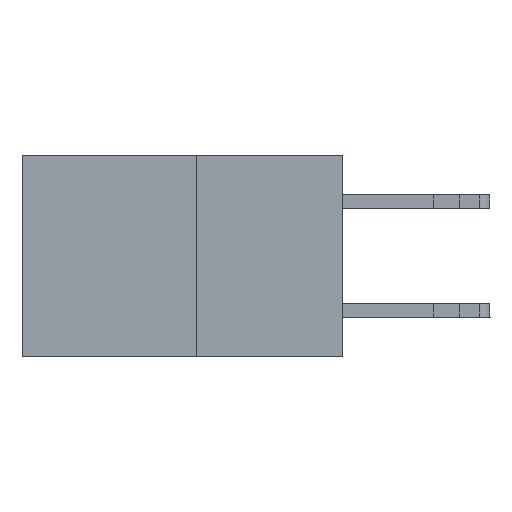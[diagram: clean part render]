
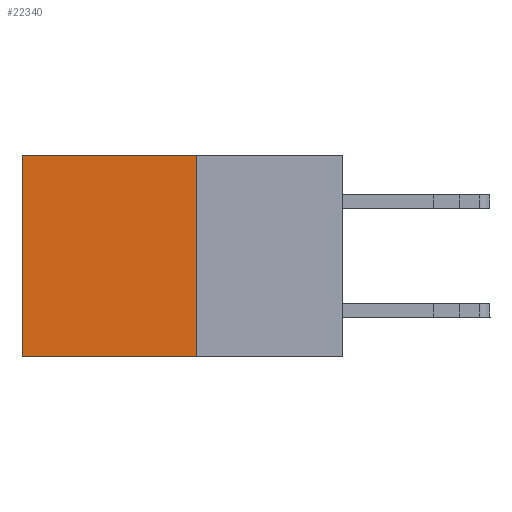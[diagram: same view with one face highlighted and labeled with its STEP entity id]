
A CAD part, left-side view. The second image highlights one B-rep face of the part: STEP entity #22340.
In plain terms, the highlighted planar face has unit normal (-1, 0, 0).
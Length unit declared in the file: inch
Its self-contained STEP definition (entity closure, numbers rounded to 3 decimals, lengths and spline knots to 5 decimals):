
#15 = FACE_OUTER_BOUND ( 'NONE', #9674, .T. ) ;
#626 = EDGE_CURVE ( 'NONE', #16173, #25570, #2988, .T. ) ;
#962 = CARTESIAN_POINT ( 'NONE',  ( 0.277, 0.27, 0. ) ) ;
#1759 = EDGE_CURVE ( 'NONE', #25570, #7474, #30136, .T. ) ;
#1913 = CARTESIAN_POINT ( 'NONE',  ( 0.277, 0.59, 0. ) ) ;
#2135 = VECTOR ( 'NONE', #17358, 39.37008 ) ;
#2988 = LINE ( 'NONE', #18882, #15824 ) ;
#3161 = ORIENTED_EDGE ( 'NONE', *, *, #626, .T. ) ;
#3325 = VECTOR ( 'NONE', #21980, 39.37008 ) ;
#5244 = CARTESIAN_POINT ( 'NONE',  ( 0.277, 0.27, -0.37 ) ) ;
#6015 = DIRECTION ( 'NONE',  ( 1., 0., 0. ) ) ;
#6571 = VECTOR ( 'NONE', #14515, 39.37008 ) ;
#6784 = CARTESIAN_POINT ( 'NONE',  ( 0.277, 0.59, -0.37 ) ) ;
#7377 = LINE ( 'NONE', #26948, #6571 ) ;
#7414 = ORIENTED_EDGE ( 'NONE', *, *, #11581, .F. ) ;
#7474 = VERTEX_POINT ( 'NONE', #6784 ) ;
#9674 = EDGE_LOOP ( 'NONE', ( #11839, #17599, #7414, #3161 ) ) ;
#11581 = EDGE_CURVE ( 'NONE', #16173, #16617, #7377, .T. ) ;
#11839 = ORIENTED_EDGE ( 'NONE', *, *, #1759, .T. ) ;
#14515 = DIRECTION ( 'NONE',  ( 0., 0., -1. ) ) ;
#14595 = AXIS2_PLACEMENT_3D ( 'NONE', #21241, #6015, #23762 ) ;
#14783 = CARTESIAN_POINT ( 'NONE',  ( 0.277, 0.27, -0.37 ) ) ;
#15747 = LINE ( 'NONE', #14783, #2135 ) ;
#15824 = VECTOR ( 'NONE', #31754, 39.37008 ) ;
#16173 = VERTEX_POINT ( 'NONE', #962 ) ;
#16617 = VERTEX_POINT ( 'NONE', #5244 ) ;
#17358 = DIRECTION ( 'NONE',  ( 0., 1., 0. ) ) ;
#17599 = ORIENTED_EDGE ( 'NONE', *, *, #20094, .F. ) ;
#18746 = PLANE ( 'NONE',  #14595 ) ;
#18759 = CARTESIAN_POINT ( 'NONE',  ( 0.277, 0.59, -0.37 ) ) ;
#18882 = CARTESIAN_POINT ( 'NONE',  ( 0.277, 0.27, 0. ) ) ;
#20094 = EDGE_CURVE ( 'NONE', #16617, #7474, #15747, .T. ) ;
#21241 = CARTESIAN_POINT ( 'NONE',  ( 0.277, 0.27, -0.37 ) ) ;
#21980 = DIRECTION ( 'NONE',  ( 0., 0., -1. ) ) ;
#22340 = ADVANCED_FACE ( 'NONE', ( #15 ), #18746, .F. ) ;
#23762 = DIRECTION ( 'NONE',  ( 0., 0., -1. ) ) ;
#25570 = VERTEX_POINT ( 'NONE', #1913 ) ;
#26948 = CARTESIAN_POINT ( 'NONE',  ( 0.277, 0.27, -0.37 ) ) ;
#30136 = LINE ( 'NONE', #18759, #3325 ) ;
#31754 = DIRECTION ( 'NONE',  ( 0., 1., 0. ) ) ;
